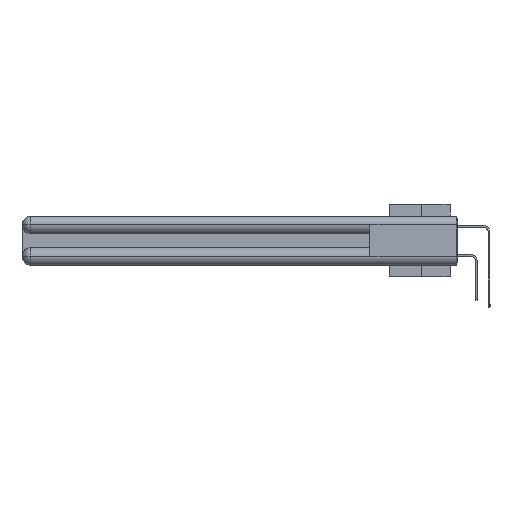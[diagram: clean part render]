
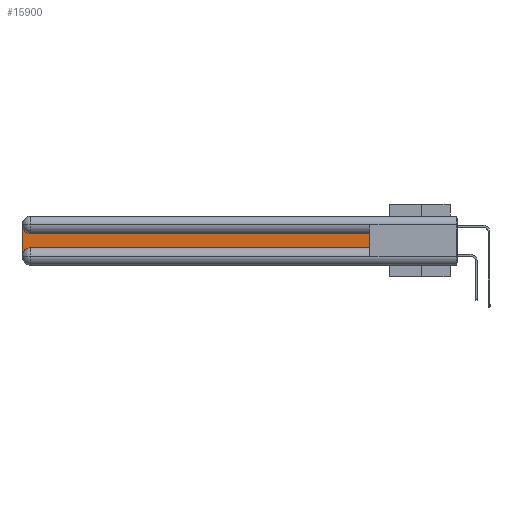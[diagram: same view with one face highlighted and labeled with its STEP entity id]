
A CAD part, left-side view. The second image highlights one B-rep face of the part: STEP entity #15900.
In plain terms, the highlighted planar face has unit normal (-1, 0, 0).
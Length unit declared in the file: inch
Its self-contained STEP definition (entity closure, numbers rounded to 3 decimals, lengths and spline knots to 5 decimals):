
#654 = EDGE_CURVE ( 'NONE', #25972, #28209, #17892, .T. ) ;
#1546 = EDGE_CURVE ( 'NONE', #8562, #37029, #14222, .T. ) ;
#1905 = ORIENTED_EDGE ( 'NONE', *, *, #18446, .T. ) ;
#2063 = DIRECTION ( 'NONE',  ( 0., 0., -1. ) ) ;
#2400 = AXIS2_PLACEMENT_3D ( 'NONE', #25753, #29026, #2063 ) ;
#3629 = CARTESIAN_POINT ( 'NONE',  ( 0.075, 3., -0.2175 ) ) ;
#4650 = VECTOR ( 'NONE', #33125, 39.37008 ) ;
#4997 = LINE ( 'NONE', #10437, #5185 ) ;
#5185 = VECTOR ( 'NONE', #37433, 39.37008 ) ;
#6642 = FACE_OUTER_BOUND ( 'NONE', #24615, .T. ) ;
#8316 = ORIENTED_EDGE ( 'NONE', *, *, #654, .T. ) ;
#8562 = VERTEX_POINT ( 'NONE', #9715 ) ;
#9176 = EDGE_CURVE ( 'NONE', #37029, #25552, #4997, .T. ) ;
#9715 = CARTESIAN_POINT ( 'NONE',  ( 0.075, 3., -0.2775 ) ) ;
#9885 = DIRECTION ( 'NONE',  ( 0., 1., 0. ) ) ;
#10117 = CARTESIAN_POINT ( 'NONE',  ( 0.075, 3., -0.1225 ) ) ;
#10437 = CARTESIAN_POINT ( 'NONE',  ( 0.075, 0.6, -0.2175 ) ) ;
#12724 = VECTOR ( 'NONE', #9885, 39.37008 ) ;
#13028 = DIRECTION ( 'NONE',  ( 0., 0., -1. ) ) ;
#13607 = CARTESIAN_POINT ( 'NONE',  ( 0.075, 2.94, -0.2775 ) ) ;
#14222 = CIRCLE ( 'NONE', #35926, 0.06 ) ;
#15900 = ADVANCED_FACE ( 'NONE', ( #6642 ), #33612, .F. ) ;
#17411 = VECTOR ( 'NONE', #23850, 39.37008 ) ;
#17892 = CIRCLE ( 'NONE', #2400, 0.06 ) ;
#18446 = EDGE_CURVE ( 'NONE', #28209, #8562, #30233, .T. ) ;
#18754 = CARTESIAN_POINT ( 'NONE',  ( 0.075, 0.6, -0.2175 ) ) ;
#18948 = LINE ( 'NONE', #18754, #4650 ) ;
#19451 = DIRECTION ( 'NONE',  ( 1., 0., 0. ) ) ;
#19820 = DIRECTION ( 'NONE',  ( 0., 0., -1. ) ) ;
#21635 = CARTESIAN_POINT ( 'NONE',  ( 0.075, 0.6, -0.2175 ) ) ;
#22120 = CARTESIAN_POINT ( 'NONE',  ( 0.075, 2.94, -0.1225 ) ) ;
#23850 = DIRECTION ( 'NONE',  ( 0., 0., -1. ) ) ;
#23854 = ORIENTED_EDGE ( 'NONE', *, *, #33498, .T. ) ;
#24615 = EDGE_LOOP ( 'NONE', ( #37251, #8316, #1905, #37299, #25456, #23854 ) ) ;
#24941 = AXIS2_PLACEMENT_3D ( 'NONE', #10117, #36921, #13028 ) ;
#25456 = ORIENTED_EDGE ( 'NONE', *, *, #9176, .T. ) ;
#25552 = VERTEX_POINT ( 'NONE', #21635 ) ;
#25753 = CARTESIAN_POINT ( 'NONE',  ( 0.075, 2.94, -0.0625 ) ) ;
#25818 = EDGE_CURVE ( 'NONE', #31693, #25972, #33577, .T. ) ;
#25972 = VERTEX_POINT ( 'NONE', #22120 ) ;
#28209 = VERTEX_POINT ( 'NONE', #28426 ) ;
#28426 = CARTESIAN_POINT ( 'NONE',  ( 0.075, 3., -0.0625 ) ) ;
#29026 = DIRECTION ( 'NONE',  ( 1., 0., 0. ) ) ;
#29597 = CARTESIAN_POINT ( 'NONE',  ( 0.075, 2.94, -0.2175 ) ) ;
#30233 = LINE ( 'NONE', #3629, #17411 ) ;
#31693 = VERTEX_POINT ( 'NONE', #35833 ) ;
#33125 = DIRECTION ( 'NONE',  ( 0., 0., 1. ) ) ;
#33211 = CARTESIAN_POINT ( 'NONE',  ( 0.075, 0.6, -0.1225 ) ) ;
#33498 = EDGE_CURVE ( 'NONE', #25552, #31693, #18948, .T. ) ;
#33577 = LINE ( 'NONE', #33211, #12724 ) ;
#33612 = PLANE ( 'NONE',  #24941 ) ;
#35833 = CARTESIAN_POINT ( 'NONE',  ( 0.075, 0.6, -0.1225 ) ) ;
#35926 = AXIS2_PLACEMENT_3D ( 'NONE', #13607, #19451, #19820 ) ;
#36921 = DIRECTION ( 'NONE',  ( 1., 0., 0. ) ) ;
#37029 = VERTEX_POINT ( 'NONE', #29597 ) ;
#37251 = ORIENTED_EDGE ( 'NONE', *, *, #25818, .T. ) ;
#37299 = ORIENTED_EDGE ( 'NONE', *, *, #1546, .T. ) ;
#37433 = DIRECTION ( 'NONE',  ( 0., -1., 0. ) ) ;
